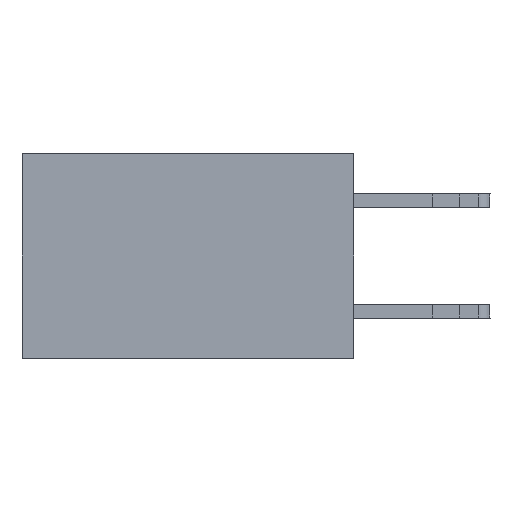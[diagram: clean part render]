
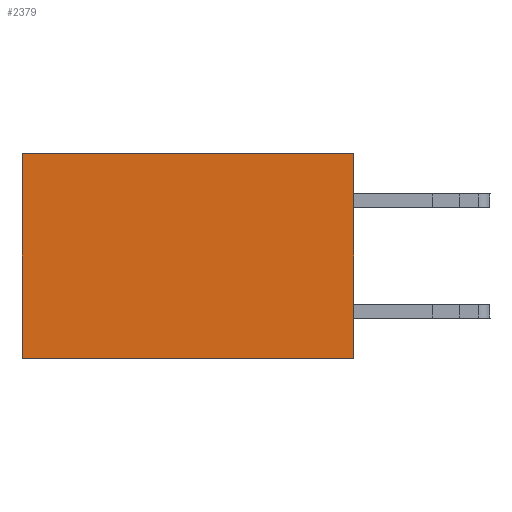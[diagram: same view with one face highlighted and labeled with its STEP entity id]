
A CAD part, left-side view. The second image highlights one B-rep face of the part: STEP entity #2379.
In plain terms, the highlighted planar face has unit normal (-1, 0, 0).
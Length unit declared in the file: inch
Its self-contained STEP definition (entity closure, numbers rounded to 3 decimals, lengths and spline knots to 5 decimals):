
#548 = LINE ( 'NONE', #22154, #19062 ) ;
#679 = CARTESIAN_POINT ( 'NONE',  ( 0.2875, 0., 0. ) ) ;
#1924 = CARTESIAN_POINT ( 'NONE',  ( 0.2875, 0., 0. ) ) ;
#2028 = VECTOR ( 'NONE', #26010, 39.37008 ) ;
#2379 = ADVANCED_FACE ( 'NONE', ( #19194 ), #7431, .F. ) ;
#3228 = CARTESIAN_POINT ( 'NONE',  ( 0.2875, 0.6, -0.37 ) ) ;
#3924 = DIRECTION ( 'NONE',  ( 0., 0., -1. ) ) ;
#4142 = EDGE_CURVE ( 'NONE', #7113, #19567, #548, .T. ) ;
#4836 = VECTOR ( 'NONE', #3924, 39.37008 ) ;
#5148 = EDGE_CURVE ( 'NONE', #11685, #25702, #26938, .T. ) ;
#5620 = ORIENTED_EDGE ( 'NONE', *, *, #25399, .F. ) ;
#7113 = VERTEX_POINT ( 'NONE', #30136 ) ;
#7431 = PLANE ( 'NONE',  #28663 ) ;
#7505 = CARTESIAN_POINT ( 'NONE',  ( 0.2875, 0., 0. ) ) ;
#7551 = DIRECTION ( 'NONE',  ( 0., 0., -1. ) ) ;
#9124 = ORIENTED_EDGE ( 'NONE', *, *, #15713, .T. ) ;
#11631 = CARTESIAN_POINT ( 'NONE',  ( 0.2875, 0., 0. ) ) ;
#11685 = VERTEX_POINT ( 'NONE', #679 ) ;
#12215 = LINE ( 'NONE', #11631, #2028 ) ;
#15025 = CARTESIAN_POINT ( 'NONE',  ( 0.2875, 0.6, 0. ) ) ;
#15713 = EDGE_CURVE ( 'NONE', #25702, #19567, #27341, .T. ) ;
#16072 = DIRECTION ( 'NONE',  ( 0., 1., 0. ) ) ;
#17513 = ORIENTED_EDGE ( 'NONE', *, *, #4142, .F. ) ;
#18732 = CARTESIAN_POINT ( 'NONE',  ( 0.2875, 0.6, 0. ) ) ;
#19062 = VECTOR ( 'NONE', #19673, 39.37008 ) ;
#19194 = FACE_OUTER_BOUND ( 'NONE', #31467, .T. ) ;
#19567 = VERTEX_POINT ( 'NONE', #3228 ) ;
#19673 = DIRECTION ( 'NONE',  ( 0., 1., 0. ) ) ;
#22154 = CARTESIAN_POINT ( 'NONE',  ( 0.2875, 0., -0.37 ) ) ;
#24467 = DIRECTION ( 'NONE',  ( 1., 0., 0. ) ) ;
#25399 = EDGE_CURVE ( 'NONE', #11685, #7113, #12215, .T. ) ;
#25702 = VERTEX_POINT ( 'NONE', #18732 ) ;
#26010 = DIRECTION ( 'NONE',  ( 0., 0., -1. ) ) ;
#26938 = LINE ( 'NONE', #7505, #36236 ) ;
#27341 = LINE ( 'NONE', #15025, #4836 ) ;
#27641 = ORIENTED_EDGE ( 'NONE', *, *, #5148, .T. ) ;
#28663 = AXIS2_PLACEMENT_3D ( 'NONE', #1924, #24467, #7551 ) ;
#30136 = CARTESIAN_POINT ( 'NONE',  ( 0.2875, 0., -0.37 ) ) ;
#31467 = EDGE_LOOP ( 'NONE', ( #9124, #17513, #5620, #27641 ) ) ;
#36236 = VECTOR ( 'NONE', #16072, 39.37008 ) ;
